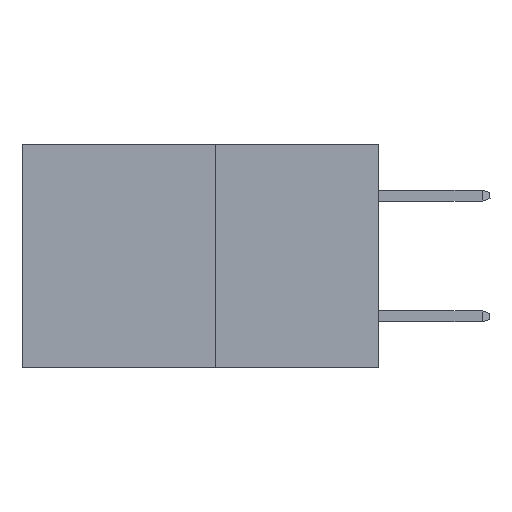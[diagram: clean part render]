
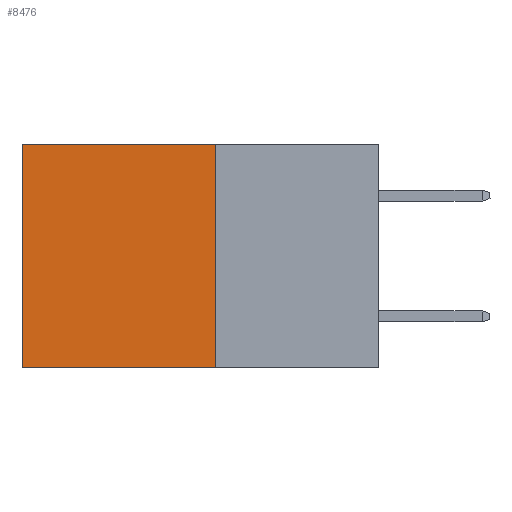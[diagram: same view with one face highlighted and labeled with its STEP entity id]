
A CAD part, left-side view. The second image highlights one B-rep face of the part: STEP entity #8476.
In plain terms, the highlighted planar face has unit normal (-1, 0, 0).
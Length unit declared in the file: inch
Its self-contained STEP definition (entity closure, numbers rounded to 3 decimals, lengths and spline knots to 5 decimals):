
#46 = VERTEX_POINT ( 'NONE', #1122 ) ;
#325 = DIRECTION ( 'NONE',  ( 0., 0., -1. ) ) ;
#333 = CARTESIAN_POINT ( 'NONE',  ( 0.277, 0.27, -0.37 ) ) ;
#466 = ORIENTED_EDGE ( 'NONE', *, *, #505, .T. ) ;
#468 = LINE ( 'NONE', #5704, #5893 ) ;
#505 = EDGE_CURVE ( 'NONE', #6310, #46, #468, .T. ) ;
#1122 = CARTESIAN_POINT ( 'NONE',  ( 0.277, 0.59, 0. ) ) ;
#1480 = CARTESIAN_POINT ( 'NONE',  ( 0.277, 0.27, -0.37 ) ) ;
#1692 = VECTOR ( 'NONE', #7262, 39.37008 ) ;
#1944 = EDGE_CURVE ( 'NONE', #6310, #3620, #5407, .T. ) ;
#1962 = CARTESIAN_POINT ( 'NONE',  ( 0.277, 0.59, -0.37 ) ) ;
#2621 = VECTOR ( 'NONE', #7605, 39.37008 ) ;
#3111 = AXIS2_PLACEMENT_3D ( 'NONE', #8639, #4568, #325 ) ;
#3454 = VECTOR ( 'NONE', #4790, 39.37008 ) ;
#3457 = CARTESIAN_POINT ( 'NONE',  ( 0.277, 0.27, -0.37 ) ) ;
#3620 = VERTEX_POINT ( 'NONE', #333 ) ;
#4027 = ORIENTED_EDGE ( 'NONE', *, *, #1944, .F. ) ;
#4568 = DIRECTION ( 'NONE',  ( 1., 0., 0. ) ) ;
#4790 = DIRECTION ( 'NONE',  ( 0., 0., -1. ) ) ;
#5147 = CARTESIAN_POINT ( 'NONE',  ( 0.277, 0.27, 0. ) ) ;
#5407 = LINE ( 'NONE', #1480, #1692 ) ;
#5410 = EDGE_CURVE ( 'NONE', #46, #6403, #7170, .T. ) ;
#5704 = CARTESIAN_POINT ( 'NONE',  ( 0.277, 0.27, 0. ) ) ;
#5893 = VECTOR ( 'NONE', #6573, 39.37008 ) ;
#5952 = CARTESIAN_POINT ( 'NONE',  ( 0.277, 0.59, -0.37 ) ) ;
#5955 = PLANE ( 'NONE',  #3111 ) ;
#6310 = VERTEX_POINT ( 'NONE', #5147 ) ;
#6403 = VERTEX_POINT ( 'NONE', #5952 ) ;
#6539 = EDGE_LOOP ( 'NONE', ( #7285, #9026, #4027, #466 ) ) ;
#6573 = DIRECTION ( 'NONE',  ( 0., 1., 0. ) ) ;
#7170 = LINE ( 'NONE', #1962, #3454 ) ;
#7262 = DIRECTION ( 'NONE',  ( 0., 0., -1. ) ) ;
#7285 = ORIENTED_EDGE ( 'NONE', *, *, #5410, .T. ) ;
#7605 = DIRECTION ( 'NONE',  ( 0., 1., 0. ) ) ;
#7941 = FACE_OUTER_BOUND ( 'NONE', #6539, .T. ) ;
#7948 = LINE ( 'NONE', #3457, #2621 ) ;
#7979 = EDGE_CURVE ( 'NONE', #3620, #6403, #7948, .T. ) ;
#8476 = ADVANCED_FACE ( 'NONE', ( #7941 ), #5955, .F. ) ;
#8639 = CARTESIAN_POINT ( 'NONE',  ( 0.277, 0.27, -0.37 ) ) ;
#9026 = ORIENTED_EDGE ( 'NONE', *, *, #7979, .F. ) ;
